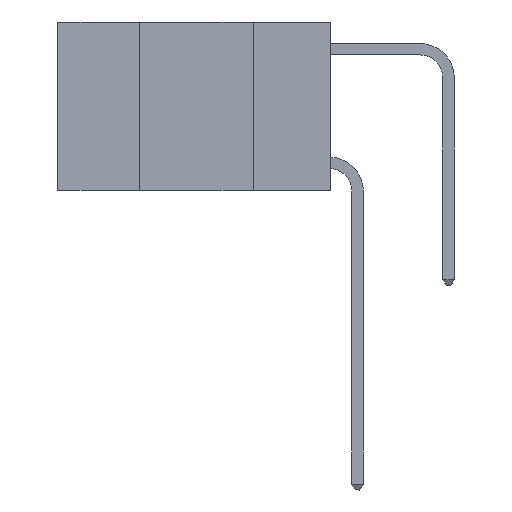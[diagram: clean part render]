
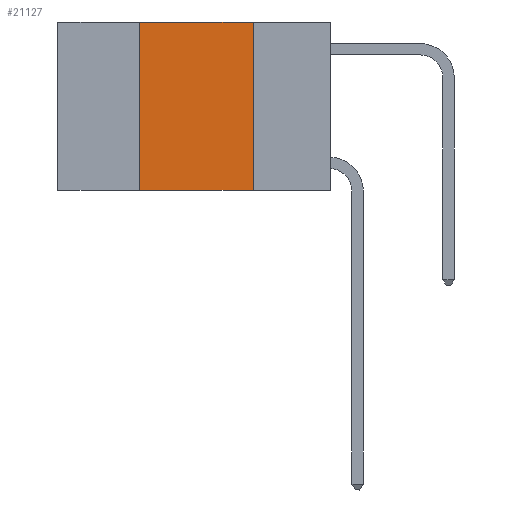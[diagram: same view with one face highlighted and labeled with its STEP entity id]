
A CAD part, left-side view. The second image highlights one B-rep face of the part: STEP entity #21127.
In plain terms, the highlighted planar face has unit normal (-1, 0, 0).
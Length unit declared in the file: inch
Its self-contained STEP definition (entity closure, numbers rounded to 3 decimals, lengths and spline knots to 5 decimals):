
#501 = LINE ( 'NONE', #8048, #3303 ) ;
#763 = VECTOR ( 'NONE', #4353, 39.37008 ) ;
#1260 = VERTEX_POINT ( 'NONE', #4515 ) ;
#1273 = FACE_OUTER_BOUND ( 'NONE', #14974, .T. ) ;
#1863 = CARTESIAN_POINT ( 'NONE',  ( 0., 0.17, 0. ) ) ;
#2986 = VERTEX_POINT ( 'NONE', #17431 ) ;
#3065 = VECTOR ( 'NONE', #13340, 39.37008 ) ;
#3303 = VECTOR ( 'NONE', #9716, 39.37008 ) ;
#3667 = LINE ( 'NONE', #21025, #11361 ) ;
#3939 = ORIENTED_EDGE ( 'NONE', *, *, #14667, .F. ) ;
#4353 = DIRECTION ( 'NONE',  ( 0., -1., 0. ) ) ;
#4451 = ORIENTED_EDGE ( 'NONE', *, *, #19471, .F. ) ;
#4515 = CARTESIAN_POINT ( 'NONE',  ( 0., 0.17, -0.37 ) ) ;
#5817 = CARTESIAN_POINT ( 'NONE',  ( 0., 0.6, 0. ) ) ;
#6478 = CARTESIAN_POINT ( 'NONE',  ( 0., 0.17, 0. ) ) ;
#6585 = VERTEX_POINT ( 'NONE', #19548 ) ;
#7484 = DIRECTION ( 'NONE',  ( 1., 0., 0. ) ) ;
#7782 = EDGE_CURVE ( 'NONE', #6585, #20756, #501, .T. ) ;
#8048 = CARTESIAN_POINT ( 'NONE',  ( 0., 0.6, 0. ) ) ;
#8296 = ORIENTED_EDGE ( 'NONE', *, *, #7782, .F. ) ;
#8727 = AXIS2_PLACEMENT_3D ( 'NONE', #5817, #7484, #18939 ) ;
#9716 = DIRECTION ( 'NONE',  ( 0., -1., 0. ) ) ;
#11242 = DIRECTION ( 'NONE',  ( 0., 0., 1. ) ) ;
#11361 = VECTOR ( 'NONE', #11242, 39.37008 ) ;
#13340 = DIRECTION ( 'NONE',  ( 0., 0., -1. ) ) ;
#13846 = LINE ( 'NONE', #14118, #763 ) ;
#14118 = CARTESIAN_POINT ( 'NONE',  ( 0., 0.6, -0.37 ) ) ;
#14667 = EDGE_CURVE ( 'NONE', #20756, #1260, #16150, .T. ) ;
#14974 = EDGE_LOOP ( 'NONE', ( #3939, #8296, #4451, #18576 ) ) ;
#15022 = EDGE_CURVE ( 'NONE', #2986, #1260, #13846, .T. ) ;
#15625 = PLANE ( 'NONE',  #8727 ) ;
#16150 = LINE ( 'NONE', #1863, #3065 ) ;
#17431 = CARTESIAN_POINT ( 'NONE',  ( 0., 0.42, -0.37 ) ) ;
#18576 = ORIENTED_EDGE ( 'NONE', *, *, #15022, .T. ) ;
#18939 = DIRECTION ( 'NONE',  ( 0., 0., -1. ) ) ;
#19471 = EDGE_CURVE ( 'NONE', #2986, #6585, #3667, .T. ) ;
#19548 = CARTESIAN_POINT ( 'NONE',  ( 0., 0.42, 0. ) ) ;
#20756 = VERTEX_POINT ( 'NONE', #6478 ) ;
#21025 = CARTESIAN_POINT ( 'NONE',  ( 0., 0.42, 0. ) ) ;
#21127 = ADVANCED_FACE ( 'NONE', ( #1273 ), #15625, .F. ) ;
